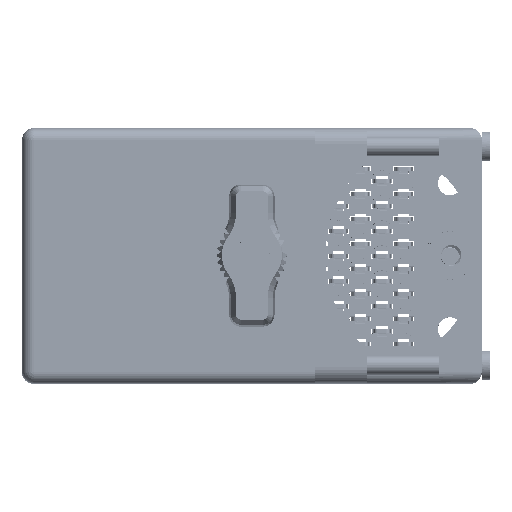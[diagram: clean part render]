
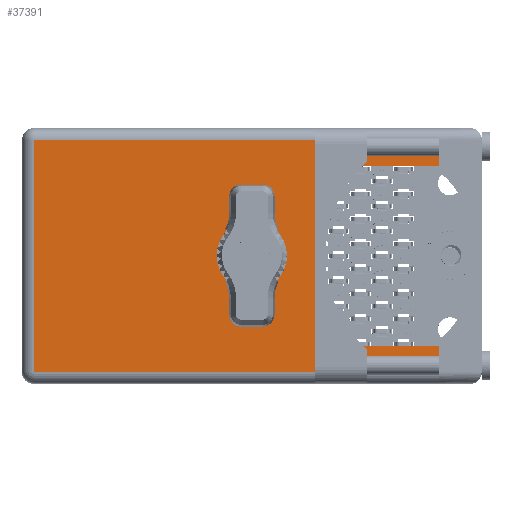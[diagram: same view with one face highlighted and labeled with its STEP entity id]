
A CAD part, top view. The second image highlights one B-rep face of the part: STEP entity #37391.
In plain terms, the highlighted face is planar.
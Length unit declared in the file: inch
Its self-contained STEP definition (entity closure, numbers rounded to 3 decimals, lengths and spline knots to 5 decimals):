
#619 = DIRECTION ( 'NONE',  ( 0., 0., 1. ) ) ;
#669 = LINE ( 'NONE', #90865, #78330 ) ;
#2842 = DIRECTION ( 'NONE',  ( -1., 0., 0. ) ) ;
#2957 = CARTESIAN_POINT ( 'NONE',  ( 1.1215, 1.93, 0.695 ) ) ;
#3598 = DIRECTION ( 'NONE',  ( 1., 0., 0. ) ) ;
#4366 = CARTESIAN_POINT ( 'NONE',  ( 1.1215, 1.93, -0.695 ) ) ;
#4819 = ORIENTED_EDGE ( 'NONE', *, *, #65458, .F. ) ;
#5940 = VECTOR ( 'NONE', #3598, 39.37008 ) ;
#6803 = DIRECTION ( 'NONE',  ( 0., 0., -1. ) ) ;
#7889 = EDGE_CURVE ( 'NONE', #14210, #102842, #22545, .T. ) ;
#8284 = VECTOR ( 'NONE', #619, 39.37008 ) ;
#9415 = CARTESIAN_POINT ( 'NONE',  ( 1.1215, 1.93, -0.54 ) ) ;
#9550 = ORIENTED_EDGE ( 'NONE', *, *, #39894, .T. ) ;
#10105 = DIRECTION ( 'NONE',  ( 0., 1., 0. ) ) ;
#11835 = DIRECTION ( 'NONE',  ( 0., 0., 1. ) ) ;
#13799 = ORIENTED_EDGE ( 'NONE', *, *, #45788, .F. ) ;
#14210 = VERTEX_POINT ( 'NONE', #96062 ) ;
#14646 = EDGE_CURVE ( 'NONE', #34260, #31235, #26946, .T. ) ;
#16101 = DIRECTION ( 'NONE',  ( 0., 1., 0. ) ) ;
#20733 = ORIENTED_EDGE ( 'NONE', *, *, #14646, .T. ) ;
#22399 = VECTOR ( 'NONE', #2842, 39.37008 ) ;
#22545 = CIRCLE ( 'NONE', #30104, 0.17 ) ;
#23804 = CARTESIAN_POINT ( 'NONE',  ( 0.4075, 1.93, -0.54 ) ) ;
#24891 = CARTESIAN_POINT ( 'NONE',  ( -1.3775, 1.93, -0.765 ) ) ;
#26946 = LINE ( 'NONE', #89663, #8284 ) ;
#27569 = VECTOR ( 'NONE', #37415, 39.37008 ) ;
#27608 = VERTEX_POINT ( 'NONE', #76978 ) ;
#29023 = CARTESIAN_POINT ( 'NONE',  ( 1.1215, 1.93, -0.765 ) ) ;
#30104 = AXIS2_PLACEMENT_3D ( 'NONE', #61080, #51711, #107355 ) ;
#30550 = LINE ( 'NONE', #48155, #5940 ) ;
#31235 = VERTEX_POINT ( 'NONE', #40175 ) ;
#32422 = VERTEX_POINT ( 'NONE', #110266 ) ;
#34260 = VERTEX_POINT ( 'NONE', #99004 ) ;
#34996 = EDGE_CURVE ( 'NONE', #102842, #14210, #38008, .T. ) ;
#35110 = VECTOR ( 'NONE', #6803, 39.37008 ) ;
#35230 = DIRECTION ( 'NONE',  ( 1., 0., 0. ) ) ;
#37391 = ADVANCED_FACE ( 'NONE', ( #71161, #69988 ), #114560, .T. ) ;
#37415 = DIRECTION ( 'NONE',  ( 0., 0., 1. ) ) ;
#38008 = CIRCLE ( 'NONE', #86655, 0.17 ) ;
#38206 = CARTESIAN_POINT ( 'NONE',  ( 0., 1.93, 0.17 ) ) ;
#39894 = EDGE_CURVE ( 'NONE', #54127, #34260, #83104, .T. ) ;
#40175 = CARTESIAN_POINT ( 'NONE',  ( -1.3075, 1.93, 0.695 ) ) ;
#41409 = CARTESIAN_POINT ( 'NONE',  ( 0.4075, 1.93, -0.54 ) ) ;
#44903 = CARTESIAN_POINT ( 'NONE',  ( 1.1215, 1.93, 0.54 ) ) ;
#45788 = EDGE_CURVE ( 'NONE', #32422, #51538, #101111, .T. ) ;
#48155 = CARTESIAN_POINT ( 'NONE',  ( 1.1215, 1.93, -0.54 ) ) ;
#48530 = CARTESIAN_POINT ( 'NONE',  ( -1.3775, 1.93, -0.695 ) ) ;
#50848 = ORIENTED_EDGE ( 'NONE', *, *, #68501, .T. ) ;
#51538 = VERTEX_POINT ( 'NONE', #2957 ) ;
#51711 = DIRECTION ( 'NONE',  ( 0., 1., 0. ) ) ;
#52149 = EDGE_LOOP ( 'NONE', ( #113532, #71438 ) ) ;
#54127 = VERTEX_POINT ( 'NONE', #4366 ) ;
#56923 = ORIENTED_EDGE ( 'NONE', *, *, #57968, .T. ) ;
#57968 = EDGE_CURVE ( 'NONE', #82726, #109786, #30550, .T. ) ;
#61080 = CARTESIAN_POINT ( 'NONE',  ( 0., 1.93, 0. ) ) ;
#62407 = DIRECTION ( 'NONE',  ( -1., 0., 0. ) ) ;
#64788 = DIRECTION ( 'NONE',  ( 0., 0., 1. ) ) ;
#65458 = EDGE_CURVE ( 'NONE', #54127, #109786, #109466, .T. ) ;
#65531 = CARTESIAN_POINT ( 'NONE',  ( 1.1215, 1.93, -0.765 ) ) ;
#66084 = VECTOR ( 'NONE', #64788, 39.37008 ) ;
#68501 = EDGE_CURVE ( 'NONE', #31235, #51538, #669, .T. ) ;
#69988 = FACE_BOUND ( 'NONE', #52149, .T. ) ;
#70068 = LINE ( 'NONE', #44903, #81807 ) ;
#71161 = FACE_OUTER_BOUND ( 'NONE', #103985, .T. ) ;
#71438 = ORIENTED_EDGE ( 'NONE', *, *, #7889, .F. ) ;
#71821 = DIRECTION ( 'NONE',  ( -1., 0., 0. ) ) ;
#76978 = CARTESIAN_POINT ( 'NONE',  ( 0.4075, 1.93, 0.54 ) ) ;
#78330 = VECTOR ( 'NONE', #35230, 39.37008 ) ;
#81807 = VECTOR ( 'NONE', #71821, 39.37008 ) ;
#82726 = VERTEX_POINT ( 'NONE', #41409 ) ;
#82848 = ORIENTED_EDGE ( 'NONE', *, *, #107540, .T. ) ;
#83104 = LINE ( 'NONE', #48530, #22399 ) ;
#86655 = AXIS2_PLACEMENT_3D ( 'NONE', #90389, #10105, #11835 ) ;
#89663 = CARTESIAN_POINT ( 'NONE',  ( -1.3075, 1.93, -0.765 ) ) ;
#90389 = CARTESIAN_POINT ( 'NONE',  ( 0., 1.93, 0. ) ) ;
#90865 = CARTESIAN_POINT ( 'NONE',  ( 1.1215, 1.93, 0.695 ) ) ;
#96062 = CARTESIAN_POINT ( 'NONE',  ( 0., 1.93, -0.17 ) ) ;
#96866 = AXIS2_PLACEMENT_3D ( 'NONE', #24891, #16101, #62407 ) ;
#99004 = CARTESIAN_POINT ( 'NONE',  ( -1.3075, 1.93, -0.695 ) ) ;
#101111 = LINE ( 'NONE', #29023, #66084 ) ;
#102842 = VERTEX_POINT ( 'NONE', #38206 ) ;
#103985 = EDGE_LOOP ( 'NONE', ( #20733, #50848, #13799, #112834, #82848, #56923, #4819, #9550 ) ) ;
#104979 = EDGE_CURVE ( 'NONE', #32422, #27608, #70068, .T. ) ;
#105260 = LINE ( 'NONE', #23804, #35110 ) ;
#107355 = DIRECTION ( 'NONE',  ( 0., 0., 1. ) ) ;
#107540 = EDGE_CURVE ( 'NONE', #27608, #82726, #105260, .T. ) ;
#109466 = LINE ( 'NONE', #65531, #27569 ) ;
#109786 = VERTEX_POINT ( 'NONE', #9415 ) ;
#110266 = CARTESIAN_POINT ( 'NONE',  ( 1.1215, 1.93, 0.54 ) ) ;
#112834 = ORIENTED_EDGE ( 'NONE', *, *, #104979, .T. ) ;
#113532 = ORIENTED_EDGE ( 'NONE', *, *, #34996, .F. ) ;
#114560 = PLANE ( 'NONE',  #96866 ) ;
